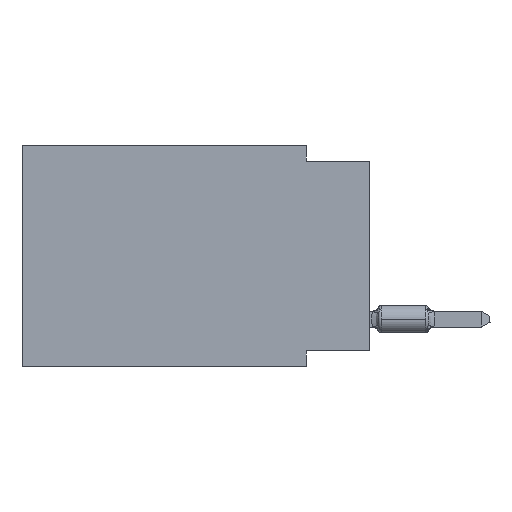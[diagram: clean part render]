
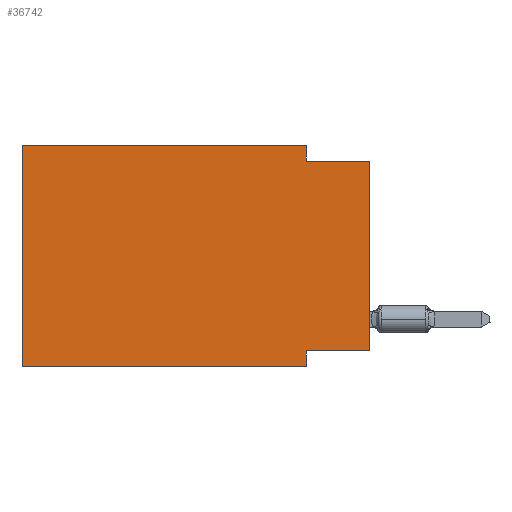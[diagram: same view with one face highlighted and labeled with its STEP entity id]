
A CAD part, left-side view. The second image highlights one B-rep face of the part: STEP entity #36742.
In plain terms, the highlighted planar face has unit normal (-1, 0, 0).
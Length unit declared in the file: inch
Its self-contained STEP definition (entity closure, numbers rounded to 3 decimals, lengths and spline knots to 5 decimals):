
#50 = ORIENTED_EDGE ( 'NONE', *, *, #37959, .F. ) ;
#285 = CARTESIAN_POINT ( 'NONE',  ( 0., 0.55, -0.35 ) ) ;
#923 = LINE ( 'NONE', #22598, #43776 ) ;
#3766 = VERTEX_POINT ( 'NONE', #11029 ) ;
#4670 = ORIENTED_EDGE ( 'NONE', *, *, #26232, .F. ) ;
#7188 = VECTOR ( 'NONE', #33960, 39.37008 ) ;
#8923 = CARTESIAN_POINT ( 'NONE',  ( 0., 0.55, 0. ) ) ;
#9081 = CARTESIAN_POINT ( 'NONE',  ( 0., 0., -0.325 ) ) ;
#9548 = DIRECTION ( 'NONE',  ( 0., 1., 0. ) ) ;
#10097 = CARTESIAN_POINT ( 'NONE',  ( 0., 0.1, -0.325 ) ) ;
#11029 = CARTESIAN_POINT ( 'NONE',  ( 0., 0.1, -0.025 ) ) ;
#11056 = ORIENTED_EDGE ( 'NONE', *, *, #37716, .F. ) ;
#12832 = AXIS2_PLACEMENT_3D ( 'NONE', #8923, #27773, #16692 ) ;
#14276 = VERTEX_POINT ( 'NONE', #27735 ) ;
#14671 = LINE ( 'NONE', #285, #17332 ) ;
#14738 = LINE ( 'NONE', #28877, #18895 ) ;
#15195 = DIRECTION ( 'NONE',  ( 0., -1., 0. ) ) ;
#15423 = VERTEX_POINT ( 'NONE', #10097 ) ;
#16467 = PLANE ( 'NONE',  #12832 ) ;
#16692 = DIRECTION ( 'NONE',  ( 0., 0., -1. ) ) ;
#17332 = VECTOR ( 'NONE', #17742, 39.37008 ) ;
#17742 = DIRECTION ( 'NONE',  ( 0., -1., 0. ) ) ;
#17890 = EDGE_CURVE ( 'NONE', #34206, #3766, #38914, .T. ) ;
#18713 = LINE ( 'NONE', #33588, #19893 ) ;
#18895 = VECTOR ( 'NONE', #25558, 39.37008 ) ;
#19893 = VECTOR ( 'NONE', #15195, 39.37008 ) ;
#20152 = VERTEX_POINT ( 'NONE', #36879 ) ;
#21220 = LINE ( 'NONE', #33721, #7188 ) ;
#22189 = DIRECTION ( 'NONE',  ( 0., -1., 0. ) ) ;
#22556 = EDGE_LOOP ( 'NONE', ( #26643, #4670, #30746, #40613, #11056, #31656, #50, #40203 ) ) ;
#22598 = CARTESIAN_POINT ( 'NONE',  ( 0., 0.55, 0. ) ) ;
#23515 = EDGE_CURVE ( 'NONE', #14276, #15423, #41616, .T. ) ;
#24206 = FACE_OUTER_BOUND ( 'NONE', #22556, .T. ) ;
#25366 = CARTESIAN_POINT ( 'NONE',  ( 0., 0.55, 0. ) ) ;
#25558 = DIRECTION ( 'NONE',  ( 0., 0., -1. ) ) ;
#25777 = EDGE_CURVE ( 'NONE', #32494, #34206, #18713, .T. ) ;
#25964 = CARTESIAN_POINT ( 'NONE',  ( 0., 0., -0.025 ) ) ;
#26232 = EDGE_CURVE ( 'NONE', #3766, #20152, #37536, .T. ) ;
#26643 = ORIENTED_EDGE ( 'NONE', *, *, #28821, .T. ) ;
#27735 = CARTESIAN_POINT ( 'NONE',  ( 0., 0., -0.325 ) ) ;
#27759 = VERTEX_POINT ( 'NONE', #41021 ) ;
#27773 = DIRECTION ( 'NONE',  ( 1., 0., 0. ) ) ;
#28821 = EDGE_CURVE ( 'NONE', #14276, #20152, #21220, .T. ) ;
#28877 = CARTESIAN_POINT ( 'NONE',  ( 0., 0.1, -0.35 ) ) ;
#29673 = VECTOR ( 'NONE', #9548, 39.37008 ) ;
#30482 = VECTOR ( 'NONE', #42207, 39.37008 ) ;
#30746 = ORIENTED_EDGE ( 'NONE', *, *, #17890, .F. ) ;
#31656 = ORIENTED_EDGE ( 'NONE', *, *, #36130, .T. ) ;
#31827 = CARTESIAN_POINT ( 'NONE',  ( 0., 0.1, 0. ) ) ;
#32402 = VERTEX_POINT ( 'NONE', #46602 ) ;
#32494 = VERTEX_POINT ( 'NONE', #25366 ) ;
#33588 = CARTESIAN_POINT ( 'NONE',  ( 0., 0.55, 0. ) ) ;
#33721 = CARTESIAN_POINT ( 'NONE',  ( 0., 0., 0. ) ) ;
#33960 = DIRECTION ( 'NONE',  ( 0., 0., 1. ) ) ;
#34206 = VERTEX_POINT ( 'NONE', #35543 ) ;
#35543 = CARTESIAN_POINT ( 'NONE',  ( 0., 0.1, 0. ) ) ;
#36130 = EDGE_CURVE ( 'NONE', #32402, #27759, #14671, .T. ) ;
#36742 = ADVANCED_FACE ( 'NONE', ( #24206 ), #16467, .F. ) ;
#36879 = CARTESIAN_POINT ( 'NONE',  ( 0., 0., -0.025 ) ) ;
#37536 = LINE ( 'NONE', #25964, #44781 ) ;
#37716 = EDGE_CURVE ( 'NONE', #32402, #32494, #923, .T. ) ;
#37959 = EDGE_CURVE ( 'NONE', #15423, #27759, #14738, .T. ) ;
#38914 = LINE ( 'NONE', #31827, #30482 ) ;
#40203 = ORIENTED_EDGE ( 'NONE', *, *, #23515, .F. ) ;
#40613 = ORIENTED_EDGE ( 'NONE', *, *, #25777, .F. ) ;
#41021 = CARTESIAN_POINT ( 'NONE',  ( 0., 0.1, -0.35 ) ) ;
#41616 = LINE ( 'NONE', #9081, #29673 ) ;
#42207 = DIRECTION ( 'NONE',  ( 0., 0., -1. ) ) ;
#43776 = VECTOR ( 'NONE', #43832, 39.37008 ) ;
#43832 = DIRECTION ( 'NONE',  ( 0., 0., 1. ) ) ;
#44781 = VECTOR ( 'NONE', #22189, 39.37008 ) ;
#46602 = CARTESIAN_POINT ( 'NONE',  ( 0., 0.55, -0.35 ) ) ;
